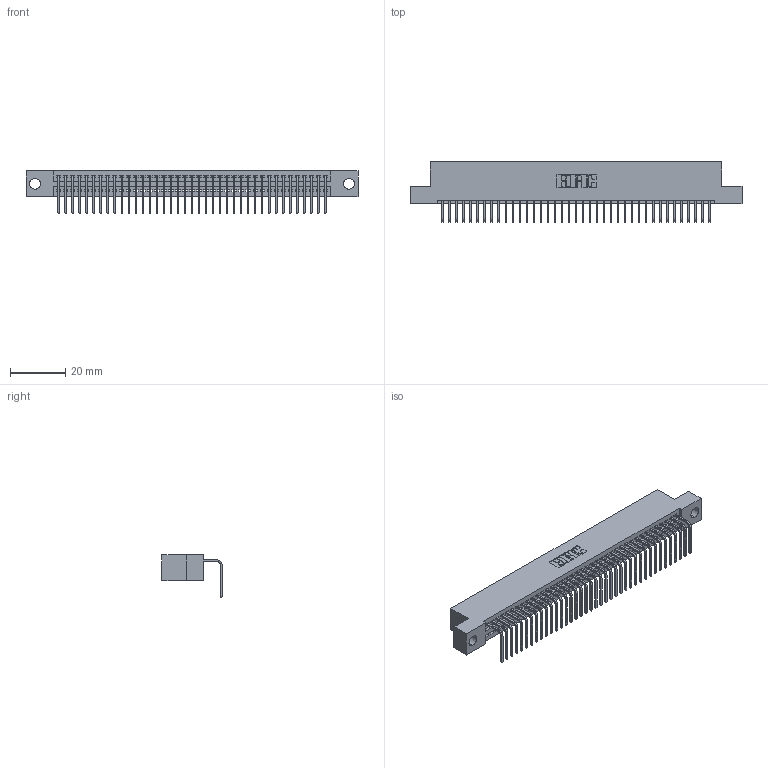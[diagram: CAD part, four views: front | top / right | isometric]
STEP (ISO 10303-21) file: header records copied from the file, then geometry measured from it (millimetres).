
FILE_DESCRIPTION (( 'STEP AP203' ), '1' );
FILE_NAME ('395-039-558-104.STEP', '2021-06-11T14:45:53', ( '' ), ( '' ), 'SwSTEP 2.0', 'SolidWorks 2020', '' );
FILE_SCHEMA (( 'CONFIG_CONTROL_DESIGN' ));
Length unit declared in the file: inch
Products named in the file (3): 345 Part_Flush Mounting Lugs - 0.156 Dia-TI; 345-292-001_558 Tail - 2; 395-039-558-104
Assembly tree (40 placements, depth 2):
  395-039-558-104
    345 Part_Flush Mounting Lugs - 0.156 Dia-TI
    345-292-001_558 Tail - 2  x39
Bounding box: 120.27 x 21.83 x 15.37 mm (x, y, z)
Volume: 11422.7 mm3; surface area: 15745 mm2
Topology: 40 solids, 40 shells, 2480 faces, 7475 edges, 4930 vertices
Faces by surface type: plane 1732, cylinder 748
Entity records: 30259 total; most frequent: CARTESIAN_POINT 5251, ORIENTED_EDGE 5222, DIRECTION 4589, EDGE_CURVE 2611, LINE 2323, VECTOR 2323, VERTEX_POINT 1738, AXIS2_PLACEMENT_3D 1133
